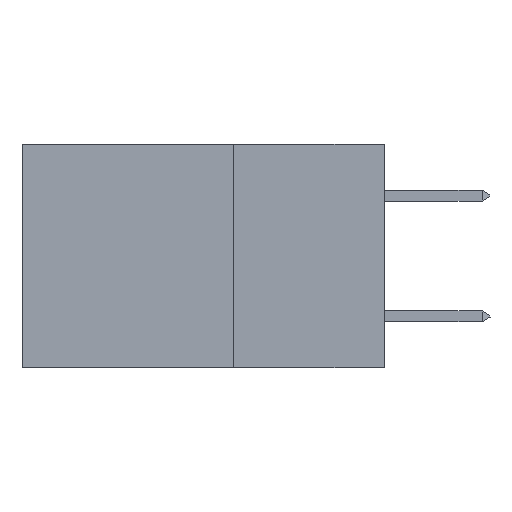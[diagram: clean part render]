
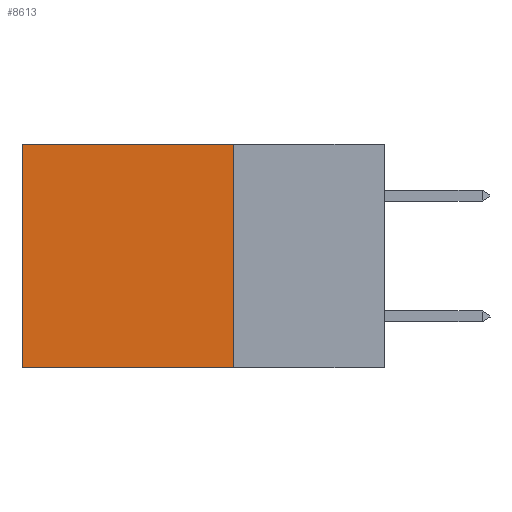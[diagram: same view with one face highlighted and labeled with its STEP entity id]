
A CAD part, left-side view. The second image highlights one B-rep face of the part: STEP entity #8613.
In plain terms, the highlighted planar face has unit normal (-1, 0, 0).
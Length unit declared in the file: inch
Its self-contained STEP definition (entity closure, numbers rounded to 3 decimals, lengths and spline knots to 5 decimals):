
#793 = CARTESIAN_POINT ( 'NONE',  ( 0.2875, 0.25, 0. ) ) ;
#814 = CARTESIAN_POINT ( 'NONE',  ( 0.2875, 0.25, 0. ) ) ;
#881 = CARTESIAN_POINT ( 'NONE',  ( 0.2875, 0.6, 0. ) ) ;
#1277 = CARTESIAN_POINT ( 'NONE',  ( 0.2875, 0.25, 0. ) ) ;
#1620 = DIRECTION ( 'NONE',  ( 1., 0., 0. ) ) ;
#1740 = VECTOR ( 'NONE', #1912, 39.37008 ) ;
#1912 = DIRECTION ( 'NONE',  ( 0., 1., 0. ) ) ;
#2014 = ORIENTED_EDGE ( 'NONE', *, *, #3748, .T. ) ;
#2331 = DIRECTION ( 'NONE',  ( 0., 0., -1. ) ) ;
#2474 = ORIENTED_EDGE ( 'NONE', *, *, #7044, .T. ) ;
#2996 = VECTOR ( 'NONE', #2331, 39.37008 ) ;
#3401 = VERTEX_POINT ( 'NONE', #3682 ) ;
#3583 = ORIENTED_EDGE ( 'NONE', *, *, #7264, .F. ) ;
#3586 = DIRECTION ( 'NONE',  ( 0., 1., 0. ) ) ;
#3682 = CARTESIAN_POINT ( 'NONE',  ( 0.2875, 0.25, -0.37 ) ) ;
#3748 = EDGE_CURVE ( 'NONE', #8679, #7071, #5236, .T. ) ;
#3873 = AXIS2_PLACEMENT_3D ( 'NONE', #814, #1620, #7020 ) ;
#4556 = VERTEX_POINT ( 'NONE', #9352 ) ;
#4657 = PLANE ( 'NONE',  #3873 ) ;
#4832 = DIRECTION ( 'NONE',  ( 0., 0., -1. ) ) ;
#5236 = LINE ( 'NONE', #1277, #7873 ) ;
#5538 = EDGE_CURVE ( 'NONE', #8679, #3401, #7965, .T. ) ;
#5907 = LINE ( 'NONE', #8335, #1740 ) ;
#6423 = CARTESIAN_POINT ( 'NONE',  ( 0.2875, 0.6, 0. ) ) ;
#6671 = VECTOR ( 'NONE', #4832, 39.37008 ) ;
#7020 = DIRECTION ( 'NONE',  ( 0., 0., -1. ) ) ;
#7044 = EDGE_CURVE ( 'NONE', #7071, #4556, #7303, .T. ) ;
#7071 = VERTEX_POINT ( 'NONE', #881 ) ;
#7264 = EDGE_CURVE ( 'NONE', #3401, #4556, #5907, .T. ) ;
#7303 = LINE ( 'NONE', #6423, #6671 ) ;
#7512 = FACE_OUTER_BOUND ( 'NONE', #8302, .T. ) ;
#7873 = VECTOR ( 'NONE', #3586, 39.37008 ) ;
#7965 = LINE ( 'NONE', #793, #2996 ) ;
#8301 = ORIENTED_EDGE ( 'NONE', *, *, #5538, .F. ) ;
#8302 = EDGE_LOOP ( 'NONE', ( #2474, #3583, #8301, #2014 ) ) ;
#8335 = CARTESIAN_POINT ( 'NONE',  ( 0.2875, 0.25, -0.37 ) ) ;
#8613 = ADVANCED_FACE ( 'NONE', ( #7512 ), #4657, .F. ) ;
#8679 = VERTEX_POINT ( 'NONE', #9495 ) ;
#9352 = CARTESIAN_POINT ( 'NONE',  ( 0.2875, 0.6, -0.37 ) ) ;
#9495 = CARTESIAN_POINT ( 'NONE',  ( 0.2875, 0.25, 0. ) ) ;
